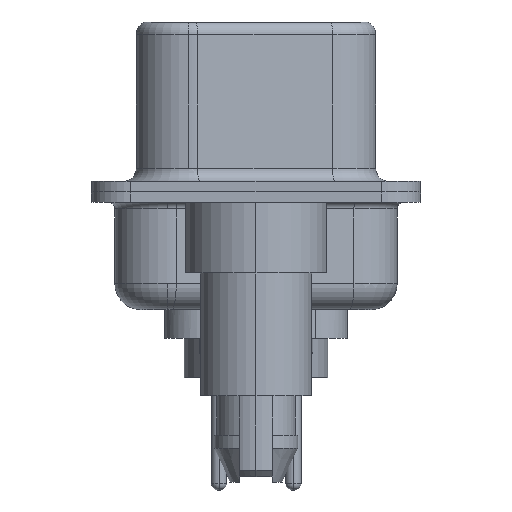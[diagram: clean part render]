
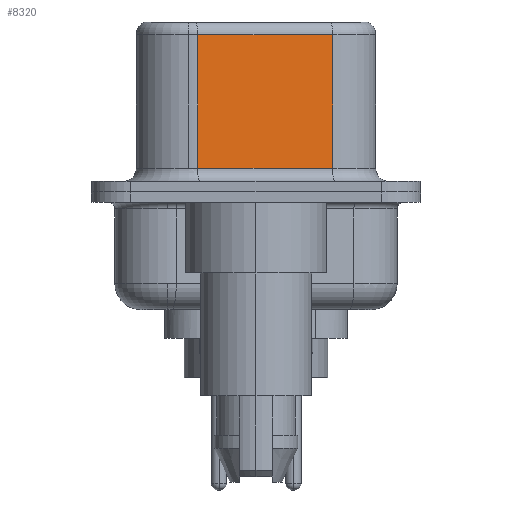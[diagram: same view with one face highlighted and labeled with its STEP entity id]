
A CAD part, left-side view. The second image highlights one B-rep face of the part: STEP entity #8320.
In plain terms, the highlighted planar face has unit normal (-0.985, -0.174, 0).
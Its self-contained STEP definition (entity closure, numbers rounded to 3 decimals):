
#375 = EDGE_LOOP ( 'NONE', ( #6313, #7719, #6620, #13403 ) ) ;
#696 = AXIS2_PLACEMENT_3D ( 'NONE', #5703, #13016, #14143 ) ;
#943 = VERTEX_POINT ( 'NONE', #8434 ) ;
#1543 = CARTESIAN_POINT ( 'NONE',  ( 4.58, -2.927, 6.02 ) ) ;
#1848 = CARTESIAN_POINT ( 'NONE',  ( 4.58, -2.927, 0.9 ) ) ;
#1923 = VECTOR ( 'NONE', #13751, 1000. ) ;
#2240 = VERTEX_POINT ( 'NONE', #1848 ) ;
#2340 = LINE ( 'NONE', #1543, #11214 ) ;
#2468 = LINE ( 'NONE', #3520, #8658 ) ;
#2824 = EDGE_CURVE ( 'NONE', #10669, #943, #13446, .T. ) ;
#3520 = CARTESIAN_POINT ( 'NONE',  ( 4.58, -2.927, 6.52 ) ) ;
#3555 = FACE_OUTER_BOUND ( 'NONE', #375, .T. ) ;
#5703 = CARTESIAN_POINT ( 'NONE',  ( 4.58, -2.927, 6.52 ) ) ;
#5802 = VERTEX_POINT ( 'NONE', #11542 ) ;
#6313 = ORIENTED_EDGE ( 'NONE', *, *, #9810, .F. ) ;
#6620 = ORIENTED_EDGE ( 'NONE', *, *, #2824, .T. ) ;
#6834 = EDGE_CURVE ( 'NONE', #943, #2240, #7794, .T. ) ;
#7095 = CARTESIAN_POINT ( 'NONE',  ( 4.58, -2.927, 0.9 ) ) ;
#7411 = VECTOR ( 'NONE', #8466, 1000. ) ;
#7719 = ORIENTED_EDGE ( 'NONE', *, *, #8164, .T. ) ;
#7794 = LINE ( 'NONE', #7095, #7411 ) ;
#8164 = EDGE_CURVE ( 'NONE', #5802, #10669, #2340, .T. ) ;
#8320 = ADVANCED_FACE ( 'NONE', ( #3555 ), #9887, .F. ) ;
#8434 = CARTESIAN_POINT ( 'NONE',  ( 3.67, 2.233, 0.9 ) ) ;
#8466 = DIRECTION ( 'NONE',  ( 0.174, -0.985, 0. ) ) ;
#8658 = VECTOR ( 'NONE', #11627, 1000. ) ;
#9810 = EDGE_CURVE ( 'NONE', #5802, #2240, #2468, .T. ) ;
#9887 = PLANE ( 'NONE',  #696 ) ;
#10669 = VERTEX_POINT ( 'NONE', #14505 ) ;
#11214 = VECTOR ( 'NONE', #12403, 1000. ) ;
#11542 = CARTESIAN_POINT ( 'NONE',  ( 4.58, -2.927, 6.02 ) ) ;
#11627 = DIRECTION ( 'NONE',  ( 0., 0., -1. ) ) ;
#12403 = DIRECTION ( 'NONE',  ( -0.174, 0.985, 0. ) ) ;
#13016 = DIRECTION ( 'NONE',  ( 0.985, 0.174, 0. ) ) ;
#13403 = ORIENTED_EDGE ( 'NONE', *, *, #6834, .T. ) ;
#13446 = LINE ( 'NONE', #14323, #1923 ) ;
#13751 = DIRECTION ( 'NONE',  ( 0., 0., -1. ) ) ;
#14143 = DIRECTION ( 'NONE',  ( -0.174, 0.985, 0. ) ) ;
#14323 = CARTESIAN_POINT ( 'NONE',  ( 3.67, 2.233, 6.52 ) ) ;
#14505 = CARTESIAN_POINT ( 'NONE',  ( 3.67, 2.233, 6.02 ) ) ;
